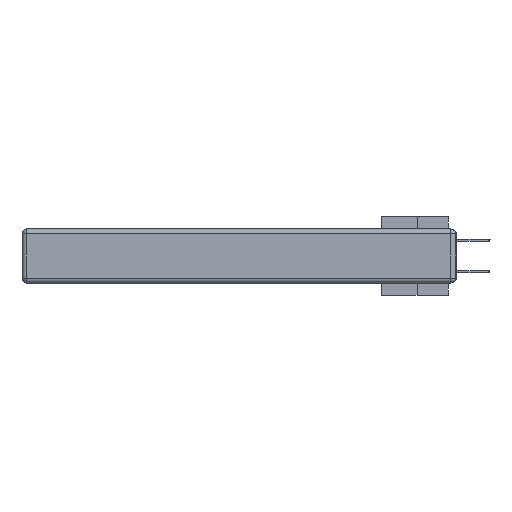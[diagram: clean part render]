
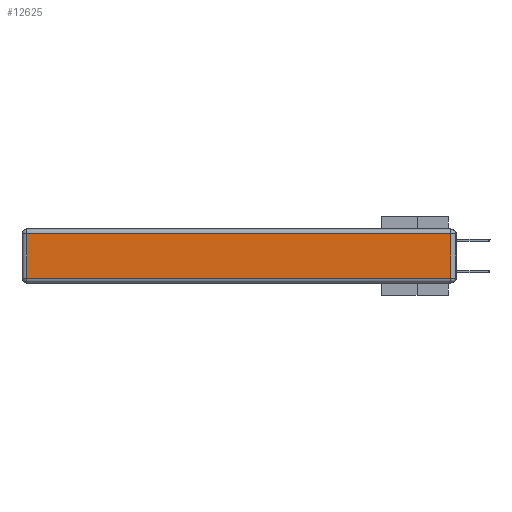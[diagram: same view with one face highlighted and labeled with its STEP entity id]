
A CAD part, left-side view. The second image highlights one B-rep face of the part: STEP entity #12625.
In plain terms, the highlighted planar face has unit normal (-1, 0, 0).
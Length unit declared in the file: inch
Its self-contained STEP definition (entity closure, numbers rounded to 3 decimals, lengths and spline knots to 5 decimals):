
#1440 = VECTOR ( 'NONE', #9713, 39.37008 ) ;
#1868 = VERTEX_POINT ( 'NONE', #34396 ) ;
#2218 = DIRECTION ( 'NONE',  ( 0., 0., -1. ) ) ;
#2243 = FACE_OUTER_BOUND ( 'NONE', #29817, .T. ) ;
#2486 = CARTESIAN_POINT ( 'NONE',  ( 0., 0., -0.343 ) ) ;
#3226 = CARTESIAN_POINT ( 'NONE',  ( 0., 0.03, -0.343 ) ) ;
#3255 = CARTESIAN_POINT ( 'NONE',  ( 0., 2.72, -0.313 ) ) ;
#4541 = EDGE_CURVE ( 'NONE', #12332, #1868, #33142, .T. ) ;
#6006 = DIRECTION ( 'NONE',  ( 0., 0., 1. ) ) ;
#6701 = LINE ( 'NONE', #15720, #31955 ) ;
#7483 = CARTESIAN_POINT ( 'NONE',  ( 0., 0., -0.313 ) ) ;
#8101 = CARTESIAN_POINT ( 'NONE',  ( 0., 0.03, -0.03 ) ) ;
#9713 = DIRECTION ( 'NONE',  ( 0., -1., 0. ) ) ;
#12332 = VERTEX_POINT ( 'NONE', #3255 ) ;
#12625 = ADVANCED_FACE ( 'NONE', ( #2243 ), #32515, .T. ) ;
#15720 = CARTESIAN_POINT ( 'NONE',  ( 0., 2.72, -0.343 ) ) ;
#16425 = DIRECTION ( 'NONE',  ( 0., 1., 0. ) ) ;
#17145 = VERTEX_POINT ( 'NONE', #8101 ) ;
#18620 = VECTOR ( 'NONE', #16425, 39.37008 ) ;
#21214 = LINE ( 'NONE', #32738, #18620 ) ;
#21614 = DIRECTION ( 'NONE',  ( -1., 0., 0. ) ) ;
#23915 = VECTOR ( 'NONE', #6006, 39.37008 ) ;
#24379 = LINE ( 'NONE', #3226, #23915 ) ;
#24396 = DIRECTION ( 'NONE',  ( 0., 0., 1. ) ) ;
#25723 = ORIENTED_EDGE ( 'NONE', *, *, #34353, .T. ) ;
#27514 = EDGE_CURVE ( 'NONE', #1868, #17145, #24379, .T. ) ;
#27943 = ORIENTED_EDGE ( 'NONE', *, *, #4541, .T. ) ;
#28723 = VERTEX_POINT ( 'NONE', #32849 ) ;
#29686 = AXIS2_PLACEMENT_3D ( 'NONE', #2486, #21614, #24396 ) ;
#29817 = EDGE_LOOP ( 'NONE', ( #27943, #34204, #25723, #34767 ) ) ;
#31955 = VECTOR ( 'NONE', #2218, 39.37008 ) ;
#32515 = PLANE ( 'NONE',  #29686 ) ;
#32738 = CARTESIAN_POINT ( 'NONE',  ( 0., 2.75, -0.03 ) ) ;
#32849 = CARTESIAN_POINT ( 'NONE',  ( 0., 2.72, -0.03 ) ) ;
#33142 = LINE ( 'NONE', #7483, #1440 ) ;
#34076 = EDGE_CURVE ( 'NONE', #28723, #12332, #6701, .T. ) ;
#34204 = ORIENTED_EDGE ( 'NONE', *, *, #27514, .T. ) ;
#34353 = EDGE_CURVE ( 'NONE', #17145, #28723, #21214, .T. ) ;
#34396 = CARTESIAN_POINT ( 'NONE',  ( 0., 0.03, -0.313 ) ) ;
#34767 = ORIENTED_EDGE ( 'NONE', *, *, #34076, .T. ) ;
